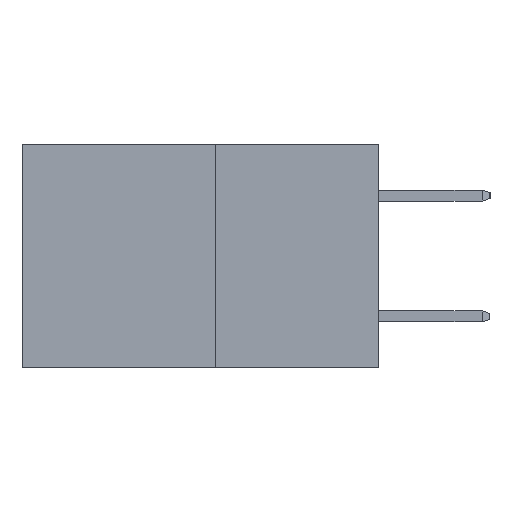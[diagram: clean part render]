
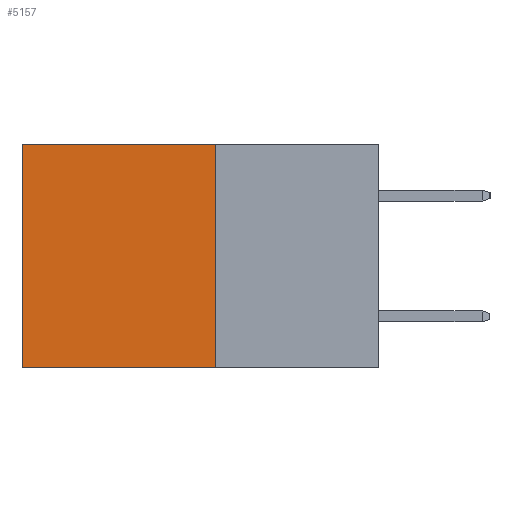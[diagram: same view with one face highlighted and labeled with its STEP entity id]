
A CAD part, left-side view. The second image highlights one B-rep face of the part: STEP entity #5157.
In plain terms, the highlighted planar face has unit normal (-1, 0, 0).
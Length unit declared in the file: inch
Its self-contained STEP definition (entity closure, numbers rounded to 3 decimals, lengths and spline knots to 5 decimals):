
#112 = EDGE_CURVE ( 'NONE', #4033, #1711, #4896, .T. ) ;
#411 = EDGE_CURVE ( 'NONE', #5709, #2527, #6078, .T. ) ;
#1364 = CARTESIAN_POINT ( 'NONE',  ( 0.277, 0.27, -0.37 ) ) ;
#1547 = CARTESIAN_POINT ( 'NONE',  ( 0.277, 0.59, 0. ) ) ;
#1711 = VERTEX_POINT ( 'NONE', #1771 ) ;
#1771 = CARTESIAN_POINT ( 'NONE',  ( 0.277, 0.59, -0.37 ) ) ;
#1906 = VECTOR ( 'NONE', #2095, 39.37008 ) ;
#2095 = DIRECTION ( 'NONE',  ( 0., 1., 0. ) ) ;
#2109 = CARTESIAN_POINT ( 'NONE',  ( 0.277, 0.27, 0. ) ) ;
#2527 = VERTEX_POINT ( 'NONE', #1547 ) ;
#2817 = FACE_OUTER_BOUND ( 'NONE', #5692, .T. ) ;
#3182 = CARTESIAN_POINT ( 'NONE',  ( 0.277, 0.27, -0.37 ) ) ;
#3353 = ORIENTED_EDGE ( 'NONE', *, *, #112, .F. ) ;
#3576 = LINE ( 'NONE', #7489, #9451 ) ;
#3615 = AXIS2_PLACEMENT_3D ( 'NONE', #1364, #9158, #4570 ) ;
#4033 = VERTEX_POINT ( 'NONE', #3182 ) ;
#4374 = EDGE_CURVE ( 'NONE', #2527, #1711, #7796, .T. ) ;
#4570 = DIRECTION ( 'NONE',  ( 0., 0., -1. ) ) ;
#4896 = LINE ( 'NONE', #8708, #5609 ) ;
#5157 = ADVANCED_FACE ( 'NONE', ( #2817 ), #8391, .F. ) ;
#5158 = CARTESIAN_POINT ( 'NONE',  ( 0.277, 0.59, -0.37 ) ) ;
#5208 = DIRECTION ( 'NONE',  ( 0., 0., -1. ) ) ;
#5609 = VECTOR ( 'NONE', #8672, 39.37008 ) ;
#5692 = EDGE_LOOP ( 'NONE', ( #9760, #3353, #7271, #8249 ) ) ;
#5709 = VERTEX_POINT ( 'NONE', #7539 ) ;
#6078 = LINE ( 'NONE', #2109, #1906 ) ;
#7271 = ORIENTED_EDGE ( 'NONE', *, *, #9313, .F. ) ;
#7489 = CARTESIAN_POINT ( 'NONE',  ( 0.277, 0.27, -0.37 ) ) ;
#7539 = CARTESIAN_POINT ( 'NONE',  ( 0.277, 0.27, 0. ) ) ;
#7796 = LINE ( 'NONE', #5158, #9586 ) ;
#8249 = ORIENTED_EDGE ( 'NONE', *, *, #411, .T. ) ;
#8391 = PLANE ( 'NONE',  #3615 ) ;
#8672 = DIRECTION ( 'NONE',  ( 0., 1., 0. ) ) ;
#8708 = CARTESIAN_POINT ( 'NONE',  ( 0.277, 0.27, -0.37 ) ) ;
#9158 = DIRECTION ( 'NONE',  ( 1., 0., 0. ) ) ;
#9313 = EDGE_CURVE ( 'NONE', #5709, #4033, #3576, .T. ) ;
#9451 = VECTOR ( 'NONE', #5208, 39.37008 ) ;
#9586 = VECTOR ( 'NONE', #9725, 39.37008 ) ;
#9725 = DIRECTION ( 'NONE',  ( 0., 0., -1. ) ) ;
#9760 = ORIENTED_EDGE ( 'NONE', *, *, #4374, .T. ) ;
